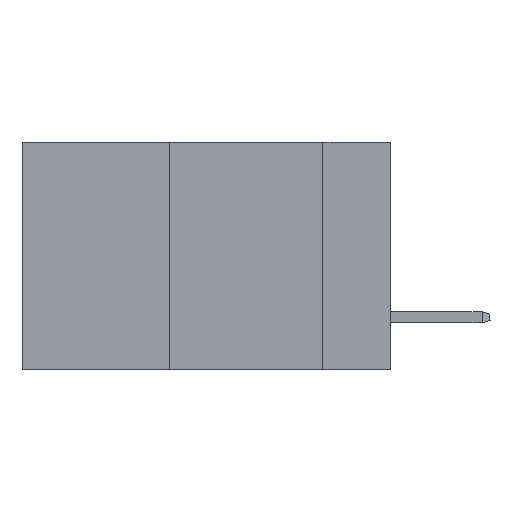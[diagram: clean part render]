
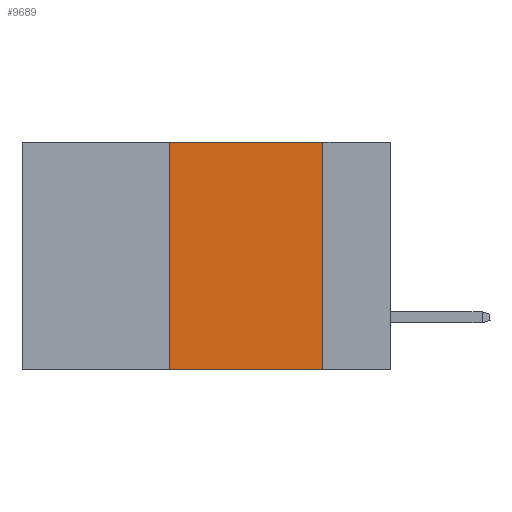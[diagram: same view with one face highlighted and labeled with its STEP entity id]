
A CAD part, left-side view. The second image highlights one B-rep face of the part: STEP entity #9689.
In plain terms, the highlighted planar face has unit normal (-1, 0, 0).
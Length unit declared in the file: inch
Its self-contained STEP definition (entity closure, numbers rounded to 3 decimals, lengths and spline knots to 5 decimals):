
#626 = CARTESIAN_POINT ( 'NONE',  ( 0., 0.36, -0.37 ) ) ;
#709 = DIRECTION ( 'NONE',  ( 0., 0., -1. ) ) ;
#1180 = EDGE_CURVE ( 'NONE', #14853, #5759, #17196, .T. ) ;
#2361 = PLANE ( 'NONE',  #5483 ) ;
#5483 = AXIS2_PLACEMENT_3D ( 'NONE', #16536, #8383, #22874 ) ;
#5759 = VERTEX_POINT ( 'NONE', #7459 ) ;
#6140 = CARTESIAN_POINT ( 'NONE',  ( 0., 0.6, 0. ) ) ;
#6482 = CARTESIAN_POINT ( 'NONE',  ( 0., 0.11, 0. ) ) ;
#7459 = CARTESIAN_POINT ( 'NONE',  ( 0., 0.11, -0.37 ) ) ;
#8383 = DIRECTION ( 'NONE',  ( 1., 0., 0. ) ) ;
#8791 = CARTESIAN_POINT ( 'NONE',  ( 0., 0.36, 0. ) ) ;
#9019 = LINE ( 'NONE', #17219, #10314 ) ;
#9689 = ADVANCED_FACE ( 'NONE', ( #23967 ), #2361, .F. ) ;
#10314 = VECTOR ( 'NONE', #709, 39.37008 ) ;
#11680 = VECTOR ( 'NONE', #17354, 39.37008 ) ;
#11686 = ORIENTED_EDGE ( 'NONE', *, *, #23628, .F. ) ;
#13079 = ORIENTED_EDGE ( 'NONE', *, *, #16909, .F. ) ;
#13283 = LINE ( 'NONE', #15709, #25600 ) ;
#13340 = CARTESIAN_POINT ( 'NONE',  ( 0., 0.6, -0.37 ) ) ;
#13789 = VERTEX_POINT ( 'NONE', #8791 ) ;
#14853 = VERTEX_POINT ( 'NONE', #626 ) ;
#15449 = ORIENTED_EDGE ( 'NONE', *, *, #15482, .F. ) ;
#15482 = EDGE_CURVE ( 'NONE', #19006, #5759, #9019, .T. ) ;
#15709 = CARTESIAN_POINT ( 'NONE',  ( 0., 0.36, 0. ) ) ;
#16038 = ORIENTED_EDGE ( 'NONE', *, *, #1180, .T. ) ;
#16175 = LINE ( 'NONE', #6140, #17185 ) ;
#16536 = CARTESIAN_POINT ( 'NONE',  ( 0., 0.6, 0. ) ) ;
#16909 = EDGE_CURVE ( 'NONE', #14853, #13789, #13283, .T. ) ;
#17185 = VECTOR ( 'NONE', #24785, 39.37008 ) ;
#17196 = LINE ( 'NONE', #13340, #11680 ) ;
#17219 = CARTESIAN_POINT ( 'NONE',  ( 0., 0.11, 0. ) ) ;
#17354 = DIRECTION ( 'NONE',  ( 0., -1., 0. ) ) ;
#17823 = DIRECTION ( 'NONE',  ( 0., 0., 1. ) ) ;
#19006 = VERTEX_POINT ( 'NONE', #6482 ) ;
#20053 = EDGE_LOOP ( 'NONE', ( #15449, #11686, #13079, #16038 ) ) ;
#22874 = DIRECTION ( 'NONE',  ( 0., 0., -1. ) ) ;
#23628 = EDGE_CURVE ( 'NONE', #13789, #19006, #16175, .T. ) ;
#23967 = FACE_OUTER_BOUND ( 'NONE', #20053, .T. ) ;
#24785 = DIRECTION ( 'NONE',  ( 0., -1., 0. ) ) ;
#25600 = VECTOR ( 'NONE', #17823, 39.37008 ) ;
